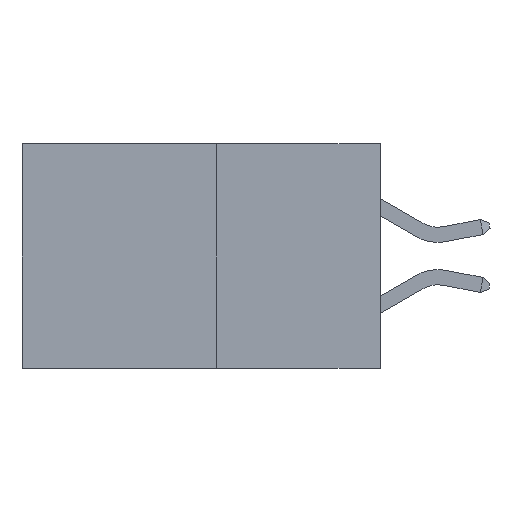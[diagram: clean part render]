
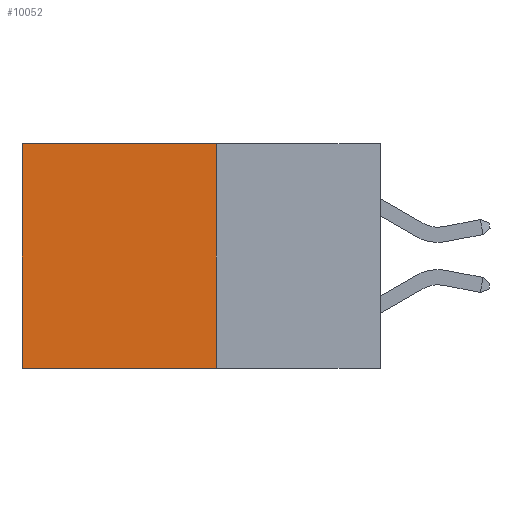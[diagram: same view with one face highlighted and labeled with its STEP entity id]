
A CAD part, left-side view. The second image highlights one B-rep face of the part: STEP entity #10052.
In plain terms, the highlighted planar face has unit normal (-1, 0, 0).
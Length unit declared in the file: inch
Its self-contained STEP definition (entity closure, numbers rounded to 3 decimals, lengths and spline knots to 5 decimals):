
#943 = VECTOR ( 'NONE', #22018, 39.37008 ) ;
#1580 = VECTOR ( 'NONE', #15313, 39.37008 ) ;
#2928 = VERTEX_POINT ( 'NONE', #7167 ) ;
#3260 = ORIENTED_EDGE ( 'NONE', *, *, #6902, .F. ) ;
#4767 = CARTESIAN_POINT ( 'NONE',  ( 0.277, 0.59, -0.37 ) ) ;
#5932 = ORIENTED_EDGE ( 'NONE', *, *, #23831, .T. ) ;
#6844 = CARTESIAN_POINT ( 'NONE',  ( 0.277, 0.27, -0.37 ) ) ;
#6902 = EDGE_CURVE ( 'NONE', #11210, #13654, #17579, .T. ) ;
#7167 = CARTESIAN_POINT ( 'NONE',  ( 0.277, 0.59, -0.37 ) ) ;
#8852 = DIRECTION ( 'NONE',  ( 0., 1., 0. ) ) ;
#8959 = CARTESIAN_POINT ( 'NONE',  ( 0.277, 0.27, -0.37 ) ) ;
#9916 = ORIENTED_EDGE ( 'NONE', *, *, #17551, .T. ) ;
#10052 = ADVANCED_FACE ( 'NONE', ( #13189 ), #21003, .F. ) ;
#10441 = AXIS2_PLACEMENT_3D ( 'NONE', #8959, #22966, #11008 ) ;
#11008 = DIRECTION ( 'NONE',  ( 0., 0., -1. ) ) ;
#11210 = VERTEX_POINT ( 'NONE', #19421 ) ;
#12682 = VECTOR ( 'NONE', #20809, 39.37008 ) ;
#13189 = FACE_OUTER_BOUND ( 'NONE', #22635, .T. ) ;
#13654 = VERTEX_POINT ( 'NONE', #23321 ) ;
#13689 = LINE ( 'NONE', #6844, #19003 ) ;
#13945 = CARTESIAN_POINT ( 'NONE',  ( 0.277, 0.59, 0. ) ) ;
#14016 = CARTESIAN_POINT ( 'NONE',  ( 0.277, 0.27, -0.37 ) ) ;
#15313 = DIRECTION ( 'NONE',  ( 0., 1., 0. ) ) ;
#15797 = VERTEX_POINT ( 'NONE', #13945 ) ;
#16140 = EDGE_CURVE ( 'NONE', #13654, #2928, #13689, .T. ) ;
#17551 = EDGE_CURVE ( 'NONE', #15797, #2928, #18665, .T. ) ;
#17579 = LINE ( 'NONE', #14016, #943 ) ;
#18665 = LINE ( 'NONE', #4767, #12682 ) ;
#19003 = VECTOR ( 'NONE', #8852, 39.37008 ) ;
#19421 = CARTESIAN_POINT ( 'NONE',  ( 0.277, 0.27, 0. ) ) ;
#20809 = DIRECTION ( 'NONE',  ( 0., 0., -1. ) ) ;
#21003 = PLANE ( 'NONE',  #10441 ) ;
#21677 = ORIENTED_EDGE ( 'NONE', *, *, #16140, .F. ) ;
#22018 = DIRECTION ( 'NONE',  ( 0., 0., -1. ) ) ;
#22635 = EDGE_LOOP ( 'NONE', ( #9916, #21677, #3260, #5932 ) ) ;
#22835 = LINE ( 'NONE', #25145, #1580 ) ;
#22966 = DIRECTION ( 'NONE',  ( 1., 0., 0. ) ) ;
#23321 = CARTESIAN_POINT ( 'NONE',  ( 0.277, 0.27, -0.37 ) ) ;
#23831 = EDGE_CURVE ( 'NONE', #11210, #15797, #22835, .T. ) ;
#25145 = CARTESIAN_POINT ( 'NONE',  ( 0.277, 0.27, 0. ) ) ;
